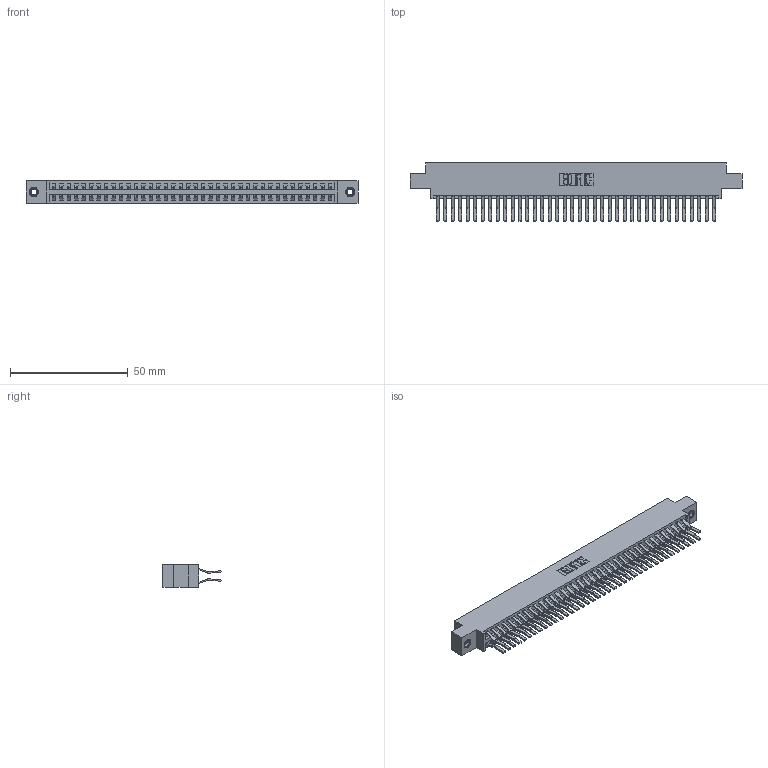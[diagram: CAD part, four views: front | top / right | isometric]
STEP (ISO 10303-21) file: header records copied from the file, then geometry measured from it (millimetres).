
FILE_DESCRIPTION (( 'STEP AP203' ), '1' );
FILE_NAME ('396-076-560-807.STEP', '2018-09-09T14:54:09', ( '' ), ( '' ), 'SwSTEP 2.0', 'SolidWorks 2016', '' );
FILE_SCHEMA (( 'CONFIG_CONTROL_DESIGN' ));
Length unit declared in the file: inch
Products named in the file (4): 346 Part_0.170 Offset - 0.156 Dia-TI; 345-292-001_560 Tail; 345-250-001_345-250-005-103; 396-076-560-807
Assembly tree (79 placements, depth 2):
  396-076-560-807
    346 Part_0.170 Offset - 0.156 Dia-TI
    345-292-001_560 Tail  x76
    345-250-001_345-250-005-103  x2
Bounding box: 141.22 x 24.78 x 9.4 mm (x, y, z)
Volume: 14070 mm3; surface area: 20819.8 mm2
Topology: 79 solids, 79 shells, 4290 faces, 12713 edges, 8366 vertices
Faces by surface type: plane 2772, cylinder 1502, cone 12, torus 4
Entity records: 26744 total; most frequent: CARTESIAN_POINT 4399, ORIENTED_EDGE 4326, DIRECTION 3957, EDGE_CURVE 2163, VECTOR 1855, LINE 1855, VERTEX_POINT 1436, AXIS2_PLACEMENT_3D 1051
